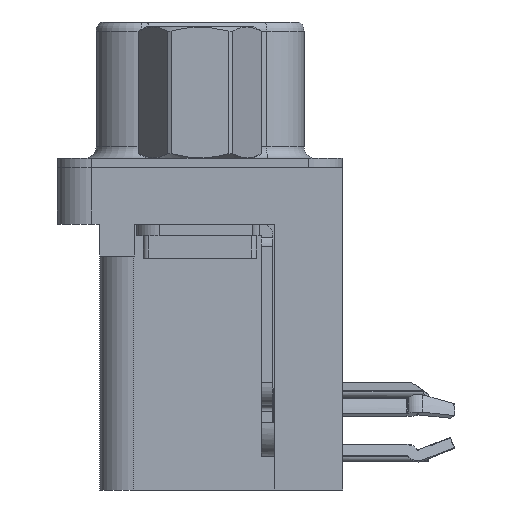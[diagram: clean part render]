
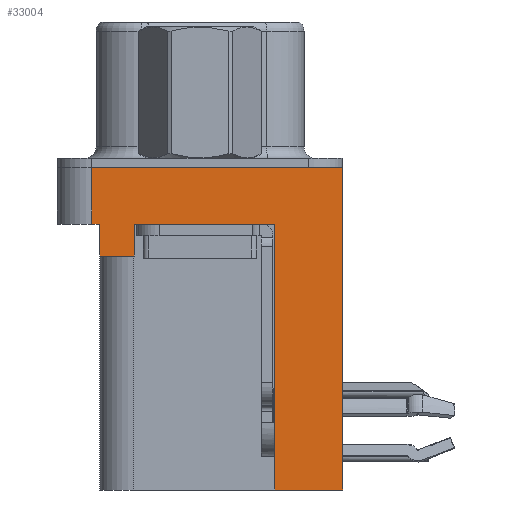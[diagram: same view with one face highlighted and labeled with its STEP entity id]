
A CAD part, left-side view. The second image highlights one B-rep face of the part: STEP entity #33004.
In plain terms, the highlighted planar face has unit normal (-1, 0, 0).
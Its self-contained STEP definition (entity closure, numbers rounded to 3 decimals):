
#456 = CARTESIAN_POINT ( 'NONE',  ( -2.91, 2.895, -2.5 ) ) ;
#684 = VERTEX_POINT ( 'NONE', #3365 ) ;
#776 = EDGE_CURVE ( 'NONE', #20776, #684, #19036, .T. ) ;
#1857 = CARTESIAN_POINT ( 'NONE',  ( -2.91, -6.275, -2.5 ) ) ;
#1920 = LINE ( 'NONE', #17105, #4032 ) ;
#2731 = ORIENTED_EDGE ( 'NONE', *, *, #23733, .T. ) ;
#3225 = ORIENTED_EDGE ( 'NONE', *, *, #776, .T. ) ;
#3365 = CARTESIAN_POINT ( 'NONE',  ( -2.91, 4.425, -2.5 ) ) ;
#3503 = EDGE_CURVE ( 'NONE', #22015, #684, #4932, .T. ) ;
#3589 = CARTESIAN_POINT ( 'NONE',  ( -2.91, -3.295, -14.2 ) ) ;
#3657 = VECTOR ( 'NONE', #25642, 1000. ) ;
#4032 = VECTOR ( 'NONE', #29629, 1000. ) ;
#4201 = CARTESIAN_POINT ( 'NONE',  ( -2.91, -6.275, 0. ) ) ;
#4307 = EDGE_CURVE ( 'NONE', #32420, #24579, #17341, .T. ) ;
#4590 = ORIENTED_EDGE ( 'NONE', *, *, #18705, .T. ) ;
#4732 = CARTESIAN_POINT ( 'NONE',  ( -2.91, 4.425, -3.9 ) ) ;
#4932 = LINE ( 'NONE', #22996, #16284 ) ;
#5935 = CARTESIAN_POINT ( 'NONE',  ( -2.91, -6.275, -2.5 ) ) ;
#5990 = EDGE_CURVE ( 'NONE', #20776, #32420, #1920, .T. ) ;
#6756 = CARTESIAN_POINT ( 'NONE',  ( -2.91, 4.775, -2.5 ) ) ;
#7073 = CARTESIAN_POINT ( 'NONE',  ( -2.91, 4.425, -3.9 ) ) ;
#7083 = DIRECTION ( 'NONE',  ( -1., 0., 0. ) ) ;
#7361 = VERTEX_POINT ( 'NONE', #10435 ) ;
#8539 = DIRECTION ( 'NONE',  ( 0., 0., 1. ) ) ;
#9419 = EDGE_CURVE ( 'NONE', #9490, #32310, #31714, .T. ) ;
#9490 = VERTEX_POINT ( 'NONE', #16989 ) ;
#10435 = CARTESIAN_POINT ( 'NONE',  ( -2.91, -3.295, -2.5 ) ) ;
#10482 = VECTOR ( 'NONE', #29173, 1000. ) ;
#10686 = VERTEX_POINT ( 'NONE', #24069 ) ;
#11059 = LINE ( 'NONE', #31680, #13789 ) ;
#11696 = EDGE_CURVE ( 'NONE', #10686, #22015, #14841, .T. ) ;
#13789 = VECTOR ( 'NONE', #8539, 1000. ) ;
#13816 = CARTESIAN_POINT ( 'NONE',  ( -2.91, -6.275, -2.5 ) ) ;
#14674 = ORIENTED_EDGE ( 'NONE', *, *, #4307, .F. ) ;
#14841 = LINE ( 'NONE', #4732, #3657 ) ;
#16050 = LINE ( 'NONE', #5935, #30791 ) ;
#16284 = VECTOR ( 'NONE', #30613, 1000. ) ;
#16989 = CARTESIAN_POINT ( 'NONE',  ( -2.91, -6.275, -14.2 ) ) ;
#17105 = CARTESIAN_POINT ( 'NONE',  ( -2.91, 4.775, -2.5 ) ) ;
#17341 = LINE ( 'NONE', #4201, #28222 ) ;
#17656 = CARTESIAN_POINT ( 'NONE',  ( -2.91, -6.275, 0. ) ) ;
#18492 = DIRECTION ( 'NONE',  ( 0., -1., 0. ) ) ;
#18705 = EDGE_CURVE ( 'NONE', #9490, #24579, #16050, .T. ) ;
#18861 = CARTESIAN_POINT ( 'NONE',  ( -2.91, -3.295, -14.2 ) ) ;
#19036 = LINE ( 'NONE', #13816, #20571 ) ;
#19246 = DIRECTION ( 'NONE',  ( 0., 0., 1. ) ) ;
#20571 = VECTOR ( 'NONE', #29355, 1000. ) ;
#20776 = VERTEX_POINT ( 'NONE', #6756 ) ;
#20952 = FACE_OUTER_BOUND ( 'NONE', #25879, .T. ) ;
#21129 = DIRECTION ( 'NONE',  ( 0., 0., 1. ) ) ;
#21176 = VERTEX_POINT ( 'NONE', #456 ) ;
#22015 = VERTEX_POINT ( 'NONE', #7073 ) ;
#22456 = VECTOR ( 'NONE', #21129, 1000. ) ;
#22996 = CARTESIAN_POINT ( 'NONE',  ( -2.91, 4.425, -3.9 ) ) ;
#23179 = ORIENTED_EDGE ( 'NONE', *, *, #11696, .F. ) ;
#23733 = EDGE_CURVE ( 'NONE', #10686, #21176, #11059, .T. ) ;
#24069 = CARTESIAN_POINT ( 'NONE',  ( -2.91, 2.895, -3.9 ) ) ;
#24071 = ORIENTED_EDGE ( 'NONE', *, *, #5990, .F. ) ;
#24579 = VERTEX_POINT ( 'NONE', #17656 ) ;
#24634 = DIRECTION ( 'NONE',  ( 0., -1., 0. ) ) ;
#24660 = AXIS2_PLACEMENT_3D ( 'NONE', #1857, #7083, #19246 ) ;
#24834 = EDGE_CURVE ( 'NONE', #21176, #7361, #31355, .T. ) ;
#25642 = DIRECTION ( 'NONE',  ( 0., 1., 0. ) ) ;
#25688 = ORIENTED_EDGE ( 'NONE', *, *, #32154, .F. ) ;
#25879 = EDGE_LOOP ( 'NONE', ( #14674, #24071, #3225, #26532, #23179, #2731, #30150, #25688, #30792, #4590 ) ) ;
#26192 = PLANE ( 'NONE',  #24660 ) ;
#26276 = CARTESIAN_POINT ( 'NONE',  ( -2.91, -6.275, -2.5 ) ) ;
#26532 = ORIENTED_EDGE ( 'NONE', *, *, #3503, .F. ) ;
#26548 = LINE ( 'NONE', #28739, #22456 ) ;
#28222 = VECTOR ( 'NONE', #24634, 1000. ) ;
#28373 = CARTESIAN_POINT ( 'NONE',  ( -2.91, 4.775, 0. ) ) ;
#28739 = CARTESIAN_POINT ( 'NONE',  ( -2.91, -3.295, -14.2 ) ) ;
#28854 = VECTOR ( 'NONE', #18492, 1000. ) ;
#29173 = DIRECTION ( 'NONE',  ( 0., 1., 0. ) ) ;
#29355 = DIRECTION ( 'NONE',  ( 0., -1., 0. ) ) ;
#29629 = DIRECTION ( 'NONE',  ( 0., 0., 1. ) ) ;
#30150 = ORIENTED_EDGE ( 'NONE', *, *, #24834, .T. ) ;
#30613 = DIRECTION ( 'NONE',  ( 0., 0., 1. ) ) ;
#30791 = VECTOR ( 'NONE', #30975, 1000. ) ;
#30792 = ORIENTED_EDGE ( 'NONE', *, *, #9419, .F. ) ;
#30975 = DIRECTION ( 'NONE',  ( 0., 0., 1. ) ) ;
#31355 = LINE ( 'NONE', #26276, #28854 ) ;
#31680 = CARTESIAN_POINT ( 'NONE',  ( -2.91, 2.895, -3.9 ) ) ;
#31714 = LINE ( 'NONE', #18861, #10482 ) ;
#32154 = EDGE_CURVE ( 'NONE', #32310, #7361, #26548, .T. ) ;
#32310 = VERTEX_POINT ( 'NONE', #3589 ) ;
#32420 = VERTEX_POINT ( 'NONE', #28373 ) ;
#33004 = ADVANCED_FACE ( 'NONE', ( #20952 ), #26192, .T. ) ;
